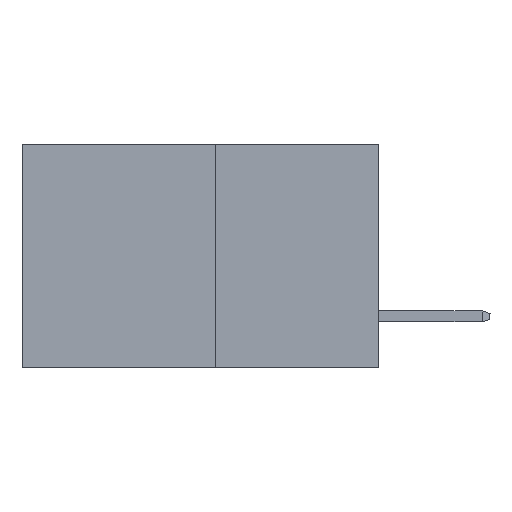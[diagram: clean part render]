
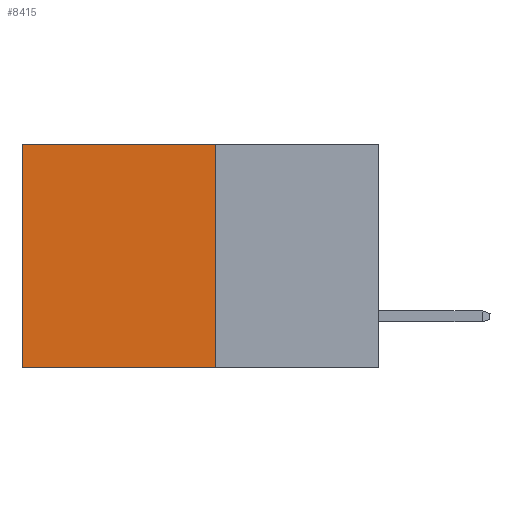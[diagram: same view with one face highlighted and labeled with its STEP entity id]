
A CAD part, left-side view. The second image highlights one B-rep face of the part: STEP entity #8415.
In plain terms, the highlighted planar face has unit normal (-1, 0, 0).
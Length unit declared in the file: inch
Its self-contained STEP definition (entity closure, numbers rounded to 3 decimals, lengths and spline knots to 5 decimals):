
#77 = EDGE_CURVE ( 'NONE', #2458, #2537, #6103, .T. ) ;
#951 = DIRECTION ( 'NONE',  ( 1., 0., 0. ) ) ;
#1093 = LINE ( 'NONE', #8941, #7938 ) ;
#1113 = CARTESIAN_POINT ( 'NONE',  ( 0.277, 0.27, -0.37 ) ) ;
#2358 = EDGE_LOOP ( 'NONE', ( #3058, #9441, #5301, #10064 ) ) ;
#2458 = VERTEX_POINT ( 'NONE', #8510 ) ;
#2537 = VERTEX_POINT ( 'NONE', #5868 ) ;
#3058 = ORIENTED_EDGE ( 'NONE', *, *, #6175, .T. ) ;
#3066 = CARTESIAN_POINT ( 'NONE',  ( 0.277, 0.27, -0.37 ) ) ;
#3081 = DIRECTION ( 'NONE',  ( 0., 1., 0. ) ) ;
#3428 = VERTEX_POINT ( 'NONE', #5932 ) ;
#3745 = EDGE_CURVE ( 'NONE', #10074, #3428, #6125, .T. ) ;
#4380 = FACE_OUTER_BOUND ( 'NONE', #2358, .T. ) ;
#5301 = ORIENTED_EDGE ( 'NONE', *, *, #5372, .F. ) ;
#5372 = EDGE_CURVE ( 'NONE', #2458, #10074, #1093, .T. ) ;
#5868 = CARTESIAN_POINT ( 'NONE',  ( 0.277, 0.59, 0. ) ) ;
#5932 = CARTESIAN_POINT ( 'NONE',  ( 0.277, 0.59, -0.37 ) ) ;
#6103 = LINE ( 'NONE', #6774, #8096 ) ;
#6125 = LINE ( 'NONE', #3066, #8653 ) ;
#6175 = EDGE_CURVE ( 'NONE', #2537, #3428, #6276, .T. ) ;
#6276 = LINE ( 'NONE', #10010, #10401 ) ;
#6404 = AXIS2_PLACEMENT_3D ( 'NONE', #11322, #951, #7270 ) ;
#6774 = CARTESIAN_POINT ( 'NONE',  ( 0.277, 0.27, 0. ) ) ;
#7270 = DIRECTION ( 'NONE',  ( 0., 0., -1. ) ) ;
#7938 = VECTOR ( 'NONE', #9719, 39.37008 ) ;
#8096 = VECTOR ( 'NONE', #11230, 39.37008 ) ;
#8415 = ADVANCED_FACE ( 'NONE', ( #4380 ), #10519, .F. ) ;
#8510 = CARTESIAN_POINT ( 'NONE',  ( 0.277, 0.27, 0. ) ) ;
#8653 = VECTOR ( 'NONE', #3081, 39.37008 ) ;
#8941 = CARTESIAN_POINT ( 'NONE',  ( 0.277, 0.27, -0.37 ) ) ;
#9441 = ORIENTED_EDGE ( 'NONE', *, *, #3745, .F. ) ;
#9719 = DIRECTION ( 'NONE',  ( 0., 0., -1. ) ) ;
#10010 = CARTESIAN_POINT ( 'NONE',  ( 0.277, 0.59, -0.37 ) ) ;
#10064 = ORIENTED_EDGE ( 'NONE', *, *, #77, .T. ) ;
#10074 = VERTEX_POINT ( 'NONE', #1113 ) ;
#10401 = VECTOR ( 'NONE', #10818, 39.37008 ) ;
#10519 = PLANE ( 'NONE',  #6404 ) ;
#10818 = DIRECTION ( 'NONE',  ( 0., 0., -1. ) ) ;
#11230 = DIRECTION ( 'NONE',  ( 0., 1., 0. ) ) ;
#11322 = CARTESIAN_POINT ( 'NONE',  ( 0.277, 0.27, -0.37 ) ) ;
